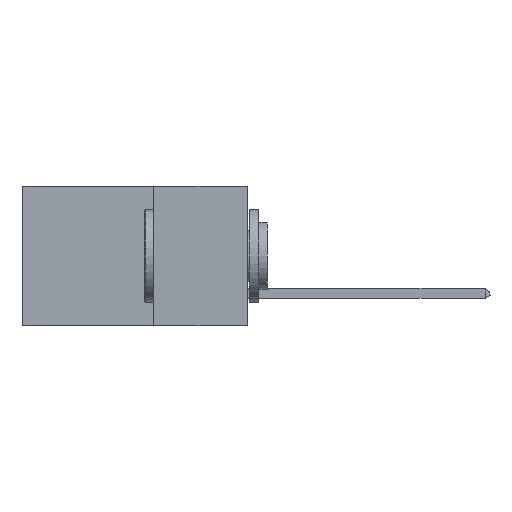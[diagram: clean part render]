
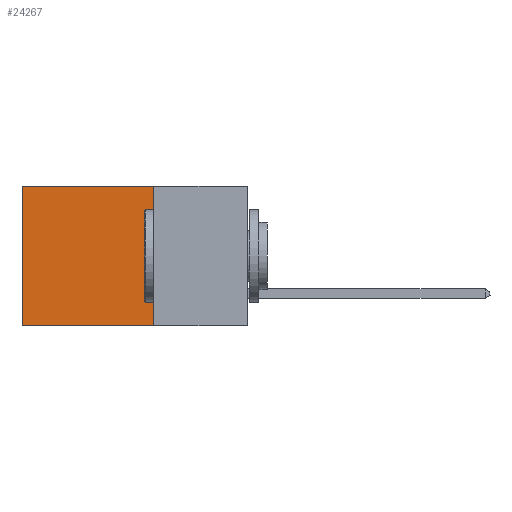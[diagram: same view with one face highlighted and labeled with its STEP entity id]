
A CAD part, left-side view. The second image highlights one B-rep face of the part: STEP entity #24267.
In plain terms, the highlighted planar face has unit normal (-1, 0, 0).
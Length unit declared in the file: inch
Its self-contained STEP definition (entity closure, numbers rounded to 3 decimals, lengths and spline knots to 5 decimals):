
#1642 = DIRECTION ( 'NONE',  ( 0., 0., -1. ) ) ;
#1860 = CARTESIAN_POINT ( 'NONE',  ( 0.298, 0.6, -0.37 ) ) ;
#2907 = CARTESIAN_POINT ( 'NONE',  ( 0.298, 0.6, 0. ) ) ;
#3090 = DIRECTION ( 'NONE',  ( 0., 1., 0. ) ) ;
#3199 = CARTESIAN_POINT ( 'NONE',  ( 0.298, 0.25, -0.37 ) ) ;
#3448 = VECTOR ( 'NONE', #24101, 39.37008 ) ;
#4045 = VERTEX_POINT ( 'NONE', #2907 ) ;
#4528 = CARTESIAN_POINT ( 'NONE',  ( 0.298, 0.25, 0. ) ) ;
#4935 = CARTESIAN_POINT ( 'NONE',  ( 0.298, 0.25, -0.37 ) ) ;
#4990 = CARTESIAN_POINT ( 'NONE',  ( 0.298, 0.25, 0. ) ) ;
#8483 = LINE ( 'NONE', #26393, #27039 ) ;
#8782 = CARTESIAN_POINT ( 'NONE',  ( 0.298, 0.6, 0. ) ) ;
#8978 = VERTEX_POINT ( 'NONE', #4935 ) ;
#10075 = PLANE ( 'NONE',  #24925 ) ;
#10645 = LINE ( 'NONE', #4528, #3448 ) ;
#12253 = LINE ( 'NONE', #3199, #14513 ) ;
#12400 = VECTOR ( 'NONE', #1642, 39.37008 ) ;
#13643 = ORIENTED_EDGE ( 'NONE', *, *, #24845, .T. ) ;
#14513 = VECTOR ( 'NONE', #3090, 39.37008 ) ;
#14520 = VERTEX_POINT ( 'NONE', #1860 ) ;
#17175 = EDGE_CURVE ( 'NONE', #8978, #14520, #12253, .T. ) ;
#17598 = ORIENTED_EDGE ( 'NONE', *, *, #29694, .T. ) ;
#18051 = EDGE_CURVE ( 'NONE', #27428, #8978, #10645, .T. ) ;
#18784 = LINE ( 'NONE', #8782, #12400 ) ;
#20112 = DIRECTION ( 'NONE',  ( 1., 0., 0. ) ) ;
#20428 = DIRECTION ( 'NONE',  ( 0., 0., -1. ) ) ;
#22895 = CARTESIAN_POINT ( 'NONE',  ( 0.298, 0.25, 0. ) ) ;
#24101 = DIRECTION ( 'NONE',  ( 0., 0., -1. ) ) ;
#24267 = ADVANCED_FACE ( 'NONE', ( #27414 ), #10075, .F. ) ;
#24301 = ORIENTED_EDGE ( 'NONE', *, *, #17175, .F. ) ;
#24845 = EDGE_CURVE ( 'NONE', #27428, #4045, #8483, .T. ) ;
#24925 = AXIS2_PLACEMENT_3D ( 'NONE', #22895, #20112, #20428 ) ;
#26393 = CARTESIAN_POINT ( 'NONE',  ( 0.298, 0.25, 0. ) ) ;
#27039 = VECTOR ( 'NONE', #30901, 39.37008 ) ;
#27414 = FACE_OUTER_BOUND ( 'NONE', #28383, .T. ) ;
#27428 = VERTEX_POINT ( 'NONE', #4990 ) ;
#28371 = ORIENTED_EDGE ( 'NONE', *, *, #18051, .F. ) ;
#28383 = EDGE_LOOP ( 'NONE', ( #17598, #24301, #28371, #13643 ) ) ;
#29694 = EDGE_CURVE ( 'NONE', #4045, #14520, #18784, .T. ) ;
#30901 = DIRECTION ( 'NONE',  ( 0., 1., 0. ) ) ;
